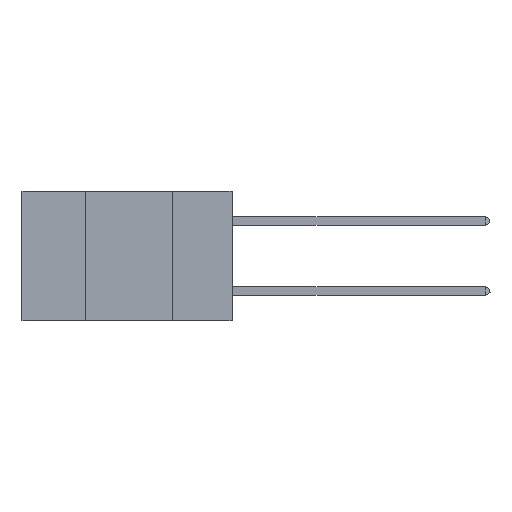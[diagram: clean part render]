
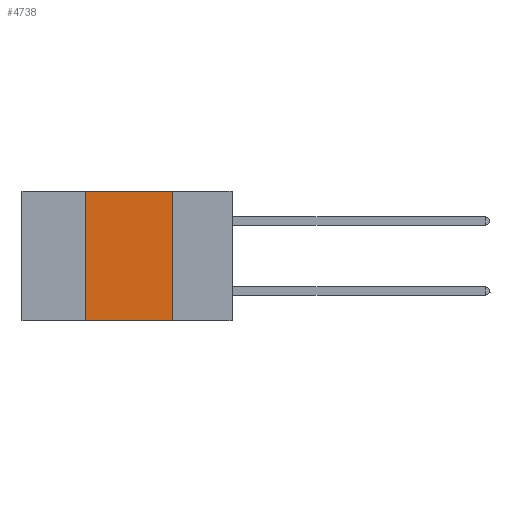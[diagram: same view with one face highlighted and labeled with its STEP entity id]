
A CAD part, left-side view. The second image highlights one B-rep face of the part: STEP entity #4738.
In plain terms, the highlighted planar face has unit normal (-1, 0, 0).
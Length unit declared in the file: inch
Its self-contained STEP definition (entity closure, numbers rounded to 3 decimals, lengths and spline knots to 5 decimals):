
#116 = DIRECTION ( 'NONE',  ( 0., 0., -1. ) ) ;
#294 = CARTESIAN_POINT ( 'NONE',  ( 0., 0.17, -0.37 ) ) ;
#1066 = LINE ( 'NONE', #15818, #5077 ) ;
#1275 = VERTEX_POINT ( 'NONE', #17662 ) ;
#1891 = VERTEX_POINT ( 'NONE', #10069 ) ;
#2028 = EDGE_CURVE ( 'NONE', #1891, #19269, #8608, .T. ) ;
#2223 = FACE_OUTER_BOUND ( 'NONE', #13533, .T. ) ;
#2810 = CARTESIAN_POINT ( 'NONE',  ( 0., 0.6, -0.37 ) ) ;
#3276 = EDGE_CURVE ( 'NONE', #19269, #19704, #20310, .T. ) ;
#3416 = EDGE_CURVE ( 'NONE', #1275, #19704, #4278, .T. ) ;
#4278 = LINE ( 'NONE', #2810, #16547 ) ;
#4727 = ORIENTED_EDGE ( 'NONE', *, *, #3416, .T. ) ;
#4738 = ADVANCED_FACE ( 'NONE', ( #2223 ), #6198, .F. ) ;
#5077 = VECTOR ( 'NONE', #6024, 39.37008 ) ;
#5657 = ORIENTED_EDGE ( 'NONE', *, *, #3276, .F. ) ;
#5798 = DIRECTION ( 'NONE',  ( 0., -1., 0. ) ) ;
#6024 = DIRECTION ( 'NONE',  ( 0., 0., 1. ) ) ;
#6198 = PLANE ( 'NONE',  #18196 ) ;
#6347 = DIRECTION ( 'NONE',  ( 0., 0., -1. ) ) ;
#7703 = ORIENTED_EDGE ( 'NONE', *, *, #2028, .F. ) ;
#8608 = LINE ( 'NONE', #16921, #12594 ) ;
#9184 = DIRECTION ( 'NONE',  ( 0., -1., 0. ) ) ;
#10069 = CARTESIAN_POINT ( 'NONE',  ( 0., 0.42, 0. ) ) ;
#11611 = ORIENTED_EDGE ( 'NONE', *, *, #17861, .F. ) ;
#11810 = VECTOR ( 'NONE', #116, 39.37008 ) ;
#12594 = VECTOR ( 'NONE', #5798, 39.37008 ) ;
#13533 = EDGE_LOOP ( 'NONE', ( #5657, #7703, #11611, #4727 ) ) ;
#14264 = DIRECTION ( 'NONE',  ( 1., 0., 0. ) ) ;
#15818 = CARTESIAN_POINT ( 'NONE',  ( 0., 0.42, 0. ) ) ;
#16547 = VECTOR ( 'NONE', #9184, 39.37008 ) ;
#16742 = CARTESIAN_POINT ( 'NONE',  ( 0., 0.17, 0. ) ) ;
#16921 = CARTESIAN_POINT ( 'NONE',  ( 0., 0.6, 0. ) ) ;
#17662 = CARTESIAN_POINT ( 'NONE',  ( 0., 0.42, -0.37 ) ) ;
#17861 = EDGE_CURVE ( 'NONE', #1275, #1891, #1066, .T. ) ;
#18108 = CARTESIAN_POINT ( 'NONE',  ( 0., 0.17, 0. ) ) ;
#18196 = AXIS2_PLACEMENT_3D ( 'NONE', #19012, #14264, #6347 ) ;
#19012 = CARTESIAN_POINT ( 'NONE',  ( 0., 0.6, 0. ) ) ;
#19269 = VERTEX_POINT ( 'NONE', #16742 ) ;
#19704 = VERTEX_POINT ( 'NONE', #294 ) ;
#20310 = LINE ( 'NONE', #18108, #11810 ) ;
